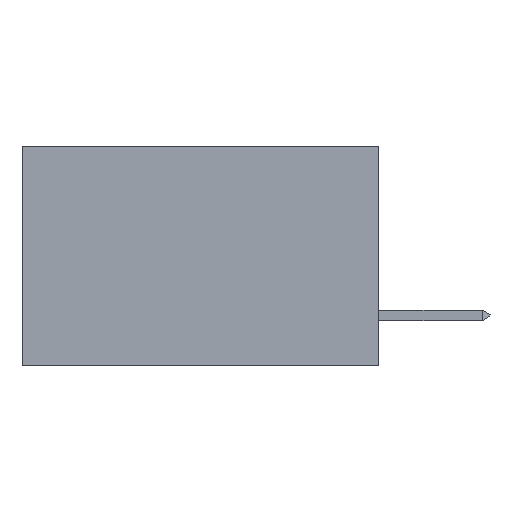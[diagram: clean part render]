
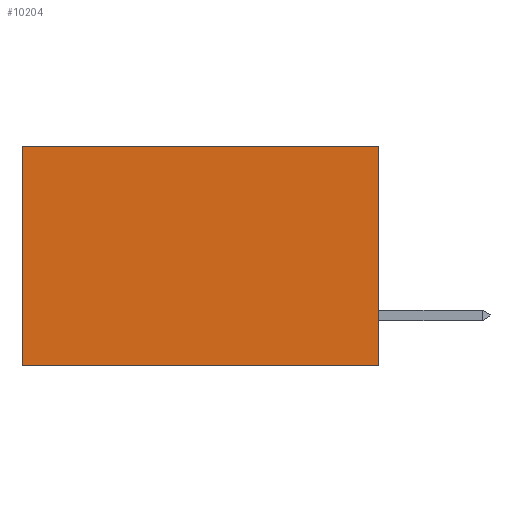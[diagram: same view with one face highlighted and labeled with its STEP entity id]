
A CAD part, left-side view. The second image highlights one B-rep face of the part: STEP entity #10204.
In plain terms, the highlighted planar face has unit normal (-1, 0, 0).
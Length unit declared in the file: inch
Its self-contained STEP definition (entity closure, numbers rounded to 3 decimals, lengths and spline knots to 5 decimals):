
#65 = LINE ( 'NONE', #3925, #4782 ) ;
#179 = DIRECTION ( 'NONE',  ( 0., 1., 0. ) ) ;
#955 = ORIENTED_EDGE ( 'NONE', *, *, #5895, .F. ) ;
#1392 = LINE ( 'NONE', #4992, #2010 ) ;
#2010 = VECTOR ( 'NONE', #179, 39.37008 ) ;
#2064 = AXIS2_PLACEMENT_3D ( 'NONE', #8533, #12395, #3718 ) ;
#2406 = ORIENTED_EDGE ( 'NONE', *, *, #5330, .F. ) ;
#2448 = DIRECTION ( 'NONE',  ( 0., 0., -1. ) ) ;
#3106 = CARTESIAN_POINT ( 'NONE',  ( 0.2615, 0., -0.37 ) ) ;
#3433 = ORIENTED_EDGE ( 'NONE', *, *, #8698, .T. ) ;
#3639 = VERTEX_POINT ( 'NONE', #3106 ) ;
#3718 = DIRECTION ( 'NONE',  ( 0., 0., -1. ) ) ;
#3759 = CARTESIAN_POINT ( 'NONE',  ( 0.2615, 0.6, -0.37 ) ) ;
#3925 = CARTESIAN_POINT ( 'NONE',  ( 0.2615, 0., 0. ) ) ;
#4445 = ORIENTED_EDGE ( 'NONE', *, *, #5964, .T. ) ;
#4782 = VECTOR ( 'NONE', #5004, 39.37008 ) ;
#4992 = CARTESIAN_POINT ( 'NONE',  ( 0.2615, 0., -0.37 ) ) ;
#5004 = DIRECTION ( 'NONE',  ( 0., 1., 0. ) ) ;
#5330 = EDGE_CURVE ( 'NONE', #3639, #6907, #1392, .T. ) ;
#5583 = VECTOR ( 'NONE', #2448, 39.37008 ) ;
#5895 = EDGE_CURVE ( 'NONE', #11225, #3639, #12008, .T. ) ;
#5964 = EDGE_CURVE ( 'NONE', #8455, #6907, #8512, .T. ) ;
#6907 = VERTEX_POINT ( 'NONE', #11627 ) ;
#6960 = CARTESIAN_POINT ( 'NONE',  ( 0.2615, 0., 0. ) ) ;
#7506 = DIRECTION ( 'NONE',  ( 0., 0., -1. ) ) ;
#7585 = FACE_OUTER_BOUND ( 'NONE', #9795, .T. ) ;
#8455 = VERTEX_POINT ( 'NONE', #11589 ) ;
#8512 = LINE ( 'NONE', #3759, #11643 ) ;
#8533 = CARTESIAN_POINT ( 'NONE',  ( 0.2615, 0., -0.37 ) ) ;
#8698 = EDGE_CURVE ( 'NONE', #11225, #8455, #65, .T. ) ;
#9795 = EDGE_LOOP ( 'NONE', ( #4445, #2406, #955, #3433 ) ) ;
#10204 = ADVANCED_FACE ( 'NONE', ( #7585 ), #10493, .F. ) ;
#10493 = PLANE ( 'NONE',  #2064 ) ;
#11225 = VERTEX_POINT ( 'NONE', #6960 ) ;
#11589 = CARTESIAN_POINT ( 'NONE',  ( 0.2615, 0.6, 0. ) ) ;
#11627 = CARTESIAN_POINT ( 'NONE',  ( 0.2615, 0.6, -0.37 ) ) ;
#11643 = VECTOR ( 'NONE', #7506, 39.37008 ) ;
#12008 = LINE ( 'NONE', #12256, #5583 ) ;
#12256 = CARTESIAN_POINT ( 'NONE',  ( 0.2615, 0., -0.37 ) ) ;
#12395 = DIRECTION ( 'NONE',  ( 1., 0., 0. ) ) ;
